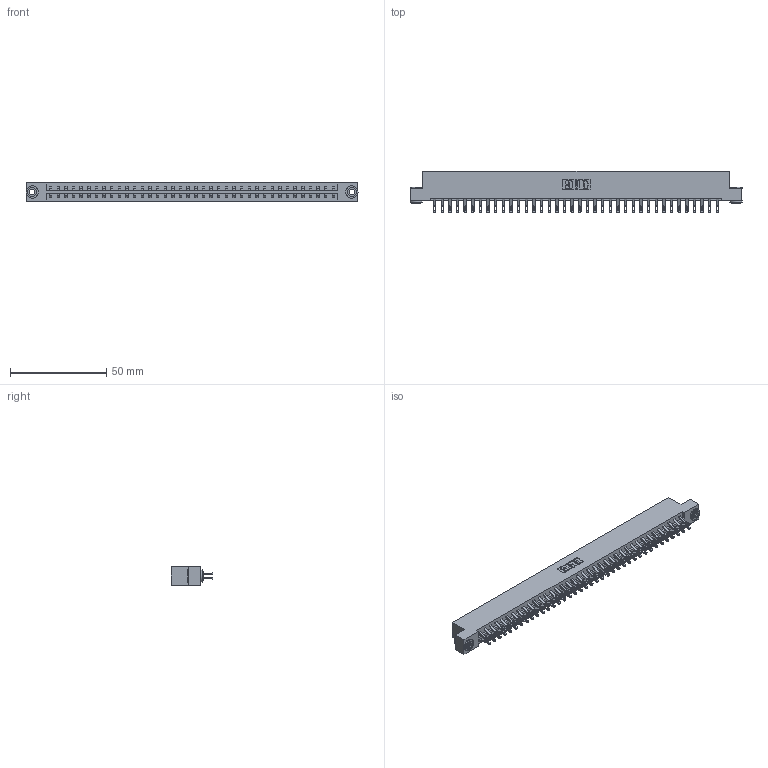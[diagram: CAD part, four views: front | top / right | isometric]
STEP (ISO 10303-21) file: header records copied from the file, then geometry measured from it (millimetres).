
FILE_DESCRIPTION (( 'STEP AP203' ), '1' );
FILE_NAME ('333-076-555-203.STEP', '2018-08-04T23:19:22', ( '' ), ( '' ), 'SwSTEP 2.0', 'SolidWorks 2016', '' );
FILE_SCHEMA (( 'CONFIG_CONTROL_DESIGN' ));
Length unit declared in the file: inch
Products named in the file (4): 345-292-001_555 Tail; 345-250-002_345-250-002-102; 333-076-555-203; 333 Part_Flush - .156 Dia - TH
Assembly tree (79 placements, depth 2):
  333-076-555-203
    333 Part_Flush - .156 Dia - TH
    345-292-001_555 Tail  x76
    345-250-002_345-250-002-102  x2
Bounding box: 172.11 x 21.47 x 9.4 mm (x, y, z)
Volume: 17773.9 mm3; surface area: 22015.5 mm2
Topology: 79 solids, 79 shells, 4560 faces, 14295 edges, 9526 vertices
Faces by surface type: plane 2664, cylinder 1888, cone 8
Entity records: 25940 total; most frequent: CARTESIAN_POINT 4315, ORIENTED_EDGE 4214, DIRECTION 3697, EDGE_CURVE 2107, LINE 1935, VECTOR 1935, VERTEX_POINT 1402, AXIS2_PLACEMENT_3D 881
